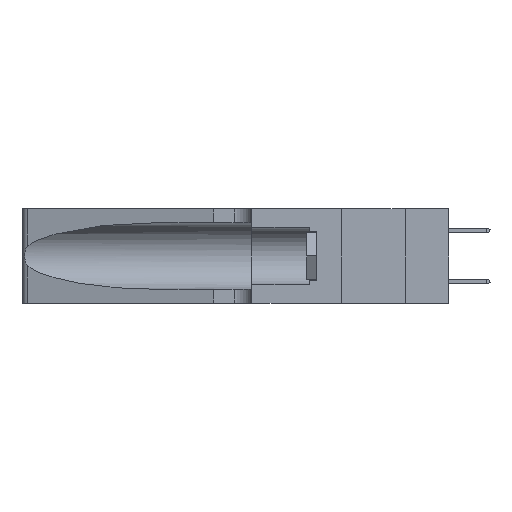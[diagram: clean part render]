
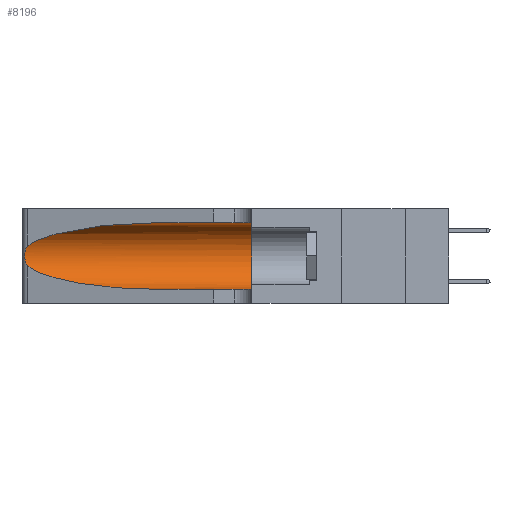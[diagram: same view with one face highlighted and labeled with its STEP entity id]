
A CAD part, left-side view. The second image highlights one B-rep face of the part: STEP entity #8196.
In plain terms, the highlighted cylindrical face has radius 3.308 mm (diameter 6.617 mm), a partial arc.
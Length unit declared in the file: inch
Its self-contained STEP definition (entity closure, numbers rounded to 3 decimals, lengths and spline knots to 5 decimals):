
#43 = B_SPLINE_CURVE_WITH_KNOTS ( 'NONE', 3,
 ( #4066, #16692, #15217, #5741, #16753, #7329, #18283, #8943, #19793, #10521, #968, #12128, #2602, #13695 ),
 .UNSPECIFIED., .F., .F.,
 ( 4, 2, 2, 2, 2, 2, 4 ),
 ( 0., 0.00027, 0.00053, 0.00107, 0.0016, 0.00187, 0.00214 ),
 .UNSPECIFIED. ) ;
#130 = EDGE_CURVE ( 'NONE', #19550, #6430, #1092, .T. ) ;
#178 = CARTESIAN_POINT ( 'NONE',  ( 0.1305, 1.61858, 0.05475 ) ) ;
#532 = VERTEX_POINT ( 'NONE', #16786 ) ;
#627 = CARTESIAN_POINT ( 'NONE',  ( 0.25487, 1.22718, 0.14631 ) ) ;
#641 = ORIENTED_EDGE ( 'NONE', *, *, #15447, .T. ) ;
#968 = CARTESIAN_POINT ( 'NONE',  ( 0.25789, 1.23486, 0.15765 ) ) ;
#1092 =( BOUNDED_CURVE ( )  B_SPLINE_CURVE ( 3, ( #627, #7506, #2194, #3667 ),
 .UNSPECIFIED., .F., .F. ) 
 B_SPLINE_CURVE_WITH_KNOTS ( ( 4, 4 ),
 ( 3.44316, 4.71239 ),
 .UNSPECIFIED. ) 
 CURVE ( )  GEOMETRIC_REPRESENTATION_ITEM ( )  RATIONAL_B_SPLINE_CURVE ( ( 1., 0.87, 0.87, 1. ) ) 
 REPRESENTATION_ITEM ( '' )  );
#1775 = EDGE_LOOP ( 'NONE', ( #641, #9698, #11055, #7011, #18526, #18722 ) ) ;
#1838 = DIRECTION ( 'NONE',  ( 0., -1., 0. ) ) ;
#2194 = CARTESIAN_POINT ( 'NONE',  ( 0.18966, 0.96281, 0.05475 ) ) ;
#2398 = CARTESIAN_POINT ( 'NONE',  ( 0.1305, 0.72297, 0.05475 ) ) ;
#2602 = CARTESIAN_POINT ( 'NONE',  ( 0.25555, 1.22993, 0.14849 ) ) ;
#3525 = CARTESIAN_POINT ( 'NONE',  ( 0.1305, 1.61858, 0.185 ) ) ;
#3667 = CARTESIAN_POINT ( 'NONE',  ( 0.1305, 0.72297, 0.05475 ) ) ;
#3779 = FACE_OUTER_BOUND ( 'NONE', #1775, .T. ) ;
#4066 = CARTESIAN_POINT ( 'NONE',  ( 0.25487, 1.22718, 0.22369 ) ) ;
#4213 = EDGE_CURVE ( 'NONE', #532, #8512, #7694, .T. ) ;
#4253 = LINE ( 'NONE', #178, #19409 ) ;
#4301 = CARTESIAN_POINT ( 'NONE',  ( 0.1305, 0.72297, 0.31525 ) ) ;
#4978 = AXIS2_PLACEMENT_3D ( 'NONE', #17155, #7753, #18668 ) ;
#5741 = CARTESIAN_POINT ( 'NONE',  ( 0.25787, 1.23484, 0.2124 ) ) ;
#5889 = CARTESIAN_POINT ( 'NONE',  ( 0.18966, 0.96281, 0.31525 ) ) ;
#6272 = AXIS2_PLACEMENT_3D ( 'NONE', #3525, #6785, #16239 ) ;
#6430 = VERTEX_POINT ( 'NONE', #2398 ) ;
#6496 = EDGE_CURVE ( 'NONE', #20104, #19550, #43, .T. ) ;
#6785 = DIRECTION ( 'NONE',  ( 0., -1., 0. ) ) ;
#7011 = ORIENTED_EDGE ( 'NONE', *, *, #9190, .T. ) ;
#7329 = CARTESIAN_POINT ( 'NONE',  ( 0.26018, 1.23835, 0.19895 ) ) ;
#7487 = CARTESIAN_POINT ( 'NONE',  ( 0.25487, 1.22718, 0.22369 ) ) ;
#7506 = CARTESIAN_POINT ( 'NONE',  ( 0.2373, 1.15595, 0.08982 ) ) ;
#7694 = LINE ( 'NONE', #15268, #11914 ) ;
#7753 = DIRECTION ( 'NONE',  ( 0., 1., 0. ) ) ;
#8024 = CIRCLE ( 'NONE', #4978, 0.13025 ) ;
#8196 = ADVANCED_FACE ( 'NONE', ( #3779 ), #15913, .F. ) ;
#8512 = VERTEX_POINT ( 'NONE', #10669 ) ;
#8943 = CARTESIAN_POINT ( 'NONE',  ( 0.26075, 1.23896, 0.178 ) ) ;
#9190 = EDGE_CURVE ( 'NONE', #6430, #17798, #4253, .T. ) ;
#9218 = CARTESIAN_POINT ( 'NONE',  ( 0.25487, 1.22718, 0.22369 ) ) ;
#9698 = ORIENTED_EDGE ( 'NONE', *, *, #6496, .T. ) ;
#10521 = CARTESIAN_POINT ( 'NONE',  ( 0.25856, 1.23593, 0.16098 ) ) ;
#10669 = CARTESIAN_POINT ( 'NONE',  ( 0.1305, 0.35, 0.31525 ) ) ;
#10824 = CARTESIAN_POINT ( 'NONE',  ( 0.25487, 1.22718, 0.14631 ) ) ;
#11055 = ORIENTED_EDGE ( 'NONE', *, *, #130, .T. ) ;
#11914 = VECTOR ( 'NONE', #16811, 39.37008 ) ;
#12128 = CARTESIAN_POINT ( 'NONE',  ( 0.25639, 1.23186, 0.15144 ) ) ;
#13695 = CARTESIAN_POINT ( 'NONE',  ( 0.25487, 1.22718, 0.14631 ) ) ;
#15217 = CARTESIAN_POINT ( 'NONE',  ( 0.25639, 1.23184, 0.21858 ) ) ;
#15268 = CARTESIAN_POINT ( 'NONE',  ( 0.1305, 1.61858, 0.31525 ) ) ;
#15447 = EDGE_CURVE ( 'NONE', #532, #20104, #16455, .T. ) ;
#15913 = CYLINDRICAL_SURFACE ( 'NONE', #6272, 0.13025 ) ;
#16239 = DIRECTION ( 'NONE',  ( 0., 0., -1. ) ) ;
#16455 =( BOUNDED_CURVE ( )  B_SPLINE_CURVE ( 3, ( #4301, #5889, #16903, #7487 ),
 .UNSPECIFIED., .F., .T. ) 
 B_SPLINE_CURVE_WITH_KNOTS ( ( 4, 4 ),
 ( 1.5708, 2.84003 ),
 .UNSPECIFIED. ) 
 CURVE ( )  GEOMETRIC_REPRESENTATION_ITEM ( )  RATIONAL_B_SPLINE_CURVE ( ( 1., 0.87, 0.87, 1. ) ) 
 REPRESENTATION_ITEM ( '' )  );
#16692 = CARTESIAN_POINT ( 'NONE',  ( 0.25555, 1.22994, 0.2215 ) ) ;
#16753 = CARTESIAN_POINT ( 'NONE',  ( 0.25854, 1.2359, 0.20912 ) ) ;
#16786 = CARTESIAN_POINT ( 'NONE',  ( 0.1305, 0.72297, 0.31525 ) ) ;
#16811 = DIRECTION ( 'NONE',  ( 0., -1., 0. ) ) ;
#16903 = CARTESIAN_POINT ( 'NONE',  ( 0.2373, 1.15595, 0.28018 ) ) ;
#17155 = CARTESIAN_POINT ( 'NONE',  ( 0.1305, 0.35, 0.185 ) ) ;
#17798 = VERTEX_POINT ( 'NONE', #19721 ) ;
#18283 = CARTESIAN_POINT ( 'NONE',  ( 0.26075, 1.23896, 0.19203 ) ) ;
#18526 = ORIENTED_EDGE ( 'NONE', *, *, #20149, .F. ) ;
#18668 = DIRECTION ( 'NONE',  ( 0., 0., 1. ) ) ;
#18722 = ORIENTED_EDGE ( 'NONE', *, *, #4213, .F. ) ;
#19409 = VECTOR ( 'NONE', #1838, 39.37008 ) ;
#19550 = VERTEX_POINT ( 'NONE', #10824 ) ;
#19721 = CARTESIAN_POINT ( 'NONE',  ( 0.1305, 0.35, 0.05475 ) ) ;
#19793 = CARTESIAN_POINT ( 'NONE',  ( 0.26017, 1.23833, 0.17102 ) ) ;
#20104 = VERTEX_POINT ( 'NONE', #9218 ) ;
#20149 = EDGE_CURVE ( 'NONE', #8512, #17798, #8024, .T. ) ;
